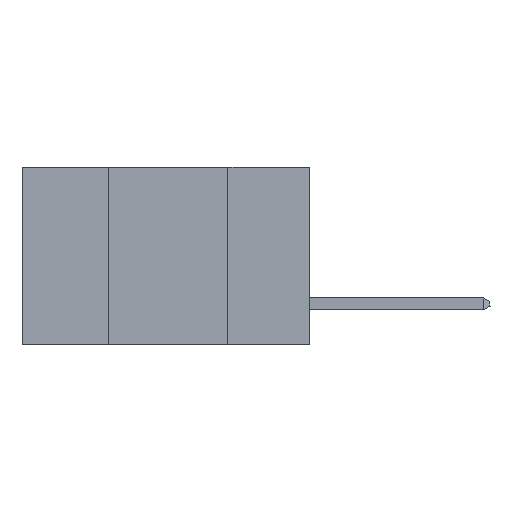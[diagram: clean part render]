
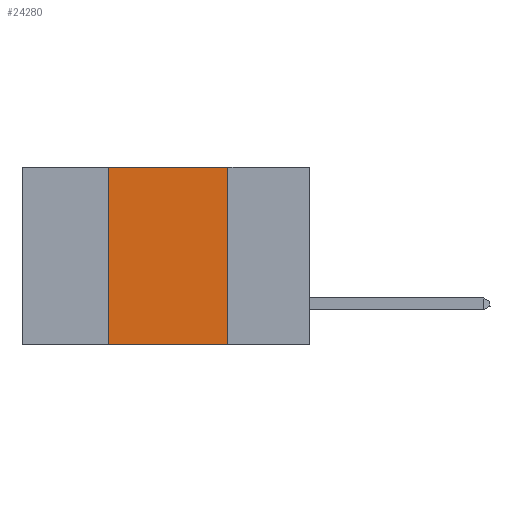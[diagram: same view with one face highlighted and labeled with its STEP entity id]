
A CAD part, left-side view. The second image highlights one B-rep face of the part: STEP entity #24280.
In plain terms, the highlighted planar face has unit normal (-1, 0, 0).
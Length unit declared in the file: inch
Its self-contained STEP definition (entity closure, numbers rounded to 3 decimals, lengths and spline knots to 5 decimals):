
#5161 = LINE ( 'NONE', #27141, #29653 ) ;
#6519 = PLANE ( 'NONE',  #17799 ) ;
#8211 = ORIENTED_EDGE ( 'NONE', *, *, #22591, .F. ) ;
#8862 = VERTEX_POINT ( 'NONE', #19344 ) ;
#11805 = CARTESIAN_POINT ( 'NONE',  ( 0., 0.17, 0. ) ) ;
#12979 = CARTESIAN_POINT ( 'NONE',  ( 0., 0.42, 0. ) ) ;
#13841 = VECTOR ( 'NONE', #30068, 39.37008 ) ;
#14303 = CARTESIAN_POINT ( 'NONE',  ( 0., 0.17, 0. ) ) ;
#14454 = ORIENTED_EDGE ( 'NONE', *, *, #17402, .F. ) ;
#15010 = EDGE_CURVE ( 'NONE', #19909, #8862, #5161, .T. ) ;
#17198 = DIRECTION ( 'NONE',  ( 0., 0., -1. ) ) ;
#17402 = EDGE_CURVE ( 'NONE', #33553, #8862, #42504, .T. ) ;
#17799 = AXIS2_PLACEMENT_3D ( 'NONE', #34437, #37724, #17198 ) ;
#18382 = VERTEX_POINT ( 'NONE', #39260 ) ;
#18915 = VECTOR ( 'NONE', #31640, 39.37008 ) ;
#18988 = EDGE_CURVE ( 'NONE', #19909, #18382, #21811, .T. ) ;
#19344 = CARTESIAN_POINT ( 'NONE',  ( 0., 0.17, -0.37 ) ) ;
#19909 = VERTEX_POINT ( 'NONE', #37571 ) ;
#21811 = LINE ( 'NONE', #12979, #13841 ) ;
#22591 = EDGE_CURVE ( 'NONE', #18382, #33553, #33257, .T. ) ;
#24280 = ADVANCED_FACE ( 'NONE', ( #25245 ), #6519, .F. ) ;
#24331 = EDGE_LOOP ( 'NONE', ( #14454, #8211, #37836, #28390 ) ) ;
#25245 = FACE_OUTER_BOUND ( 'NONE', #24331, .T. ) ;
#25879 = DIRECTION ( 'NONE',  ( 0., 0., -1. ) ) ;
#27141 = CARTESIAN_POINT ( 'NONE',  ( 0., 0.6, -0.37 ) ) ;
#28390 = ORIENTED_EDGE ( 'NONE', *, *, #15010, .T. ) ;
#29653 = VECTOR ( 'NONE', #30464, 39.37008 ) ;
#30068 = DIRECTION ( 'NONE',  ( 0., 0., 1. ) ) ;
#30464 = DIRECTION ( 'NONE',  ( 0., -1., 0. ) ) ;
#31640 = DIRECTION ( 'NONE',  ( 0., -1., 0. ) ) ;
#33257 = LINE ( 'NONE', #34932, #18915 ) ;
#33553 = VERTEX_POINT ( 'NONE', #14303 ) ;
#34437 = CARTESIAN_POINT ( 'NONE',  ( 0., 0.6, 0. ) ) ;
#34907 = VECTOR ( 'NONE', #25879, 39.37008 ) ;
#34932 = CARTESIAN_POINT ( 'NONE',  ( 0., 0.6, 0. ) ) ;
#37571 = CARTESIAN_POINT ( 'NONE',  ( 0., 0.42, -0.37 ) ) ;
#37724 = DIRECTION ( 'NONE',  ( 1., 0., 0. ) ) ;
#37836 = ORIENTED_EDGE ( 'NONE', *, *, #18988, .F. ) ;
#39260 = CARTESIAN_POINT ( 'NONE',  ( 0., 0.42, 0. ) ) ;
#42504 = LINE ( 'NONE', #11805, #34907 ) ;
